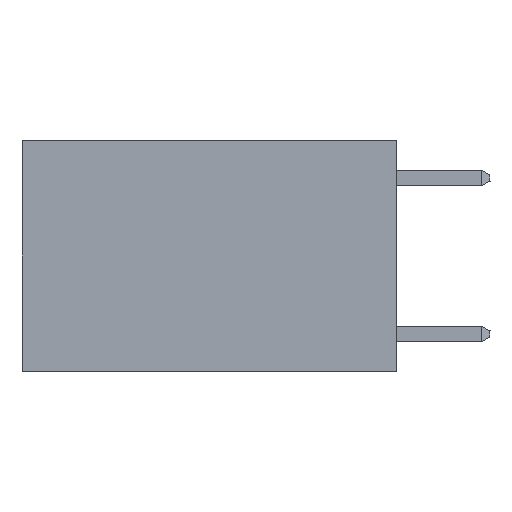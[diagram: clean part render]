
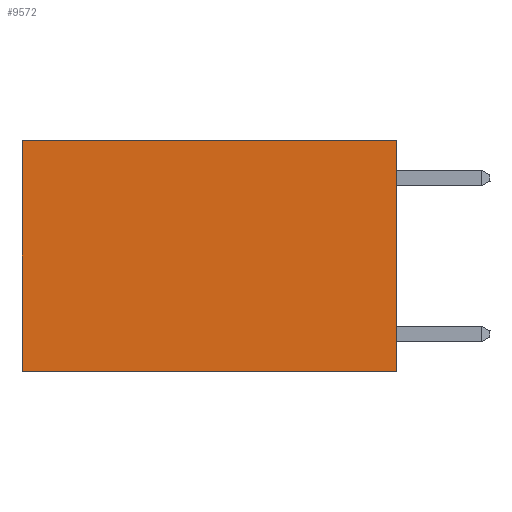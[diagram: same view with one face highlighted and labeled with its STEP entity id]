
A CAD part, left-side view. The second image highlights one B-rep face of the part: STEP entity #9572.
In plain terms, the highlighted planar face has unit normal (-1, 0, 0).
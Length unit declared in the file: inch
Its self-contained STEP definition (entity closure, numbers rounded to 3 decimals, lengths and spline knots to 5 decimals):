
#372 = AXIS2_PLACEMENT_3D ( 'NONE', #7763, #3931, #9325 ) ;
#789 = PLANE ( 'NONE',  #372 ) ;
#928 = VECTOR ( 'NONE', #5296, 39.37008 ) ;
#1417 = LINE ( 'NONE', #4960, #7265 ) ;
#1515 = DIRECTION ( 'NONE',  ( 0., 0., -1. ) ) ;
#1988 = EDGE_CURVE ( 'NONE', #8974, #9910, #1417, .T. ) ;
#2112 = ORIENTED_EDGE ( 'NONE', *, *, #9275, .T. ) ;
#2153 = ORIENTED_EDGE ( 'NONE', *, *, #1988, .F. ) ;
#2228 = CARTESIAN_POINT ( 'NONE',  ( 0.2625, 0., 0. ) ) ;
#2533 = ORIENTED_EDGE ( 'NONE', *, *, #3265, .F. ) ;
#3031 = CARTESIAN_POINT ( 'NONE',  ( 0.2625, 0.6, 0. ) ) ;
#3128 = CARTESIAN_POINT ( 'NONE',  ( 0.2625, 0., 0. ) ) ;
#3265 = EDGE_CURVE ( 'NONE', #4108, #8974, #7003, .T. ) ;
#3326 = CARTESIAN_POINT ( 'NONE',  ( 0.2625, 0., 0. ) ) ;
#3596 = ORIENTED_EDGE ( 'NONE', *, *, #8333, .T. ) ;
#3817 = CARTESIAN_POINT ( 'NONE',  ( 0.2625, 0.6, 0. ) ) ;
#3931 = DIRECTION ( 'NONE',  ( 1., 0., 0. ) ) ;
#4091 = VERTEX_POINT ( 'NONE', #3031 ) ;
#4108 = VERTEX_POINT ( 'NONE', #3128 ) ;
#4630 = EDGE_LOOP ( 'NONE', ( #2112, #2153, #2533, #3596 ) ) ;
#4957 = VECTOR ( 'NONE', #1515, 39.37008 ) ;
#4960 = CARTESIAN_POINT ( 'NONE',  ( 0.2625, 0., -0.37 ) ) ;
#5061 = DIRECTION ( 'NONE',  ( 0., 1., 0. ) ) ;
#5296 = DIRECTION ( 'NONE',  ( 0., 0., -1. ) ) ;
#5359 = LINE ( 'NONE', #3326, #9255 ) ;
#5758 = CARTESIAN_POINT ( 'NONE',  ( 0.2625, 0., -0.37 ) ) ;
#6661 = LINE ( 'NONE', #3817, #4957 ) ;
#7003 = LINE ( 'NONE', #2228, #928 ) ;
#7265 = VECTOR ( 'NONE', #5061, 39.37008 ) ;
#7274 = CARTESIAN_POINT ( 'NONE',  ( 0.2625, 0.6, -0.37 ) ) ;
#7763 = CARTESIAN_POINT ( 'NONE',  ( 0.2625, 0., 0. ) ) ;
#8151 = DIRECTION ( 'NONE',  ( 0., 1., 0. ) ) ;
#8333 = EDGE_CURVE ( 'NONE', #4108, #4091, #5359, .T. ) ;
#8974 = VERTEX_POINT ( 'NONE', #5758 ) ;
#9234 = FACE_OUTER_BOUND ( 'NONE', #4630, .T. ) ;
#9255 = VECTOR ( 'NONE', #8151, 39.37008 ) ;
#9275 = EDGE_CURVE ( 'NONE', #4091, #9910, #6661, .T. ) ;
#9325 = DIRECTION ( 'NONE',  ( 0., 0., -1. ) ) ;
#9572 = ADVANCED_FACE ( 'NONE', ( #9234 ), #789, .F. ) ;
#9910 = VERTEX_POINT ( 'NONE', #7274 ) ;
